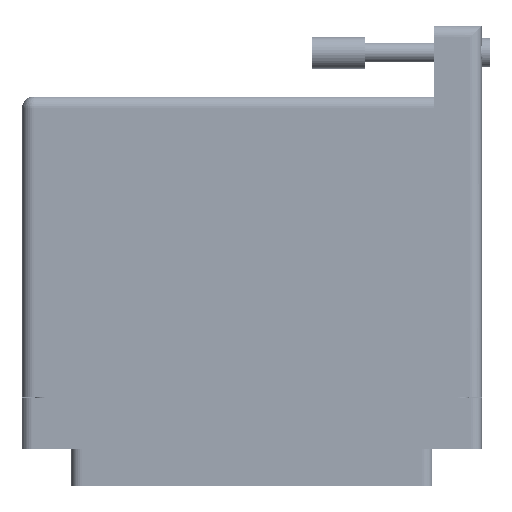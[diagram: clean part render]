
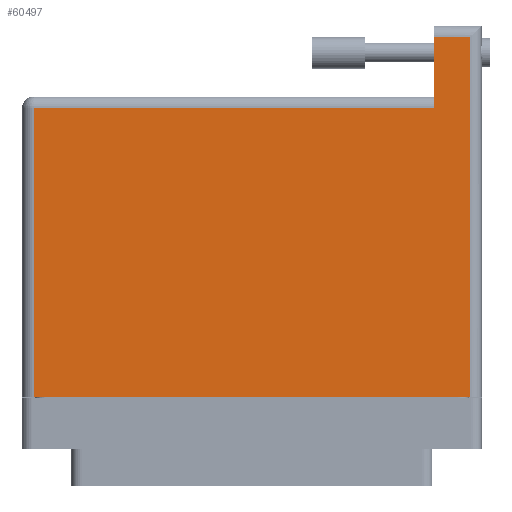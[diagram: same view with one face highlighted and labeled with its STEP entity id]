
A CAD part, front view. The second image highlights one B-rep face of the part: STEP entity #60497.
In plain terms, the highlighted face is planar.
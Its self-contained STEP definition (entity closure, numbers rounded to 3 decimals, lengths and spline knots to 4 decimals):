
#1102 = CARTESIAN_POINT ( 'NONE',  ( -1.359, 1.675, 0.617 ) ) ;
#1421 = LINE ( 'NONE', #1966, #57320 ) ;
#1966 = CARTESIAN_POINT ( 'NONE',  ( 1.079, 2.095, 0.617 ) ) ;
#2111 = FACE_OUTER_BOUND ( 'NONE', #41996, .T. ) ;
#6260 = VERTEX_POINT ( 'NONE', #32739 ) ;
#8278 = VERTEX_POINT ( 'NONE', #10705 ) ;
#10705 = CARTESIAN_POINT ( 'NONE',  ( -1.289, 1.605, 0.617 ) ) ;
#12804 = VECTOR ( 'NONE', #33574, 39.3701 ) ;
#13091 = DIRECTION ( 'NONE',  ( -1., 0., 0. ) ) ;
#14640 = VECTOR ( 'NONE', #34641, 39.3701 ) ;
#15283 = ORIENTED_EDGE ( 'NONE', *, *, #44509, .T. ) ;
#16572 = CARTESIAN_POINT ( 'NONE',  ( 1.289, -0.1, 0.617 ) ) ;
#18814 = ORIENTED_EDGE ( 'NONE', *, *, #52891, .T. ) ;
#19305 = VECTOR ( 'NONE', #24328, 39.3701 ) ;
#19913 = VERTEX_POINT ( 'NONE', #67257 ) ;
#22695 = LINE ( 'NONE', #39496, #19305 ) ;
#23028 = DIRECTION ( 'NONE',  ( 0., -1., 0. ) ) ;
#24328 = DIRECTION ( 'NONE',  ( 1., 0., 0. ) ) ;
#27177 = EDGE_CURVE ( 'NONE', #19913, #6260, #61173, .T. ) ;
#30400 = ORIENTED_EDGE ( 'NONE', *, *, #69777, .T. ) ;
#31073 = VERTEX_POINT ( 'NONE', #16572 ) ;
#32739 = CARTESIAN_POINT ( 'NONE',  ( 1.079, 2.025, 0.617 ) ) ;
#33574 = DIRECTION ( 'NONE',  ( 0., 1., 0. ) ) ;
#34641 = DIRECTION ( 'NONE',  ( -1., 0., 0. ) ) ;
#35326 = VERTEX_POINT ( 'NONE', #38211 ) ;
#38211 = CARTESIAN_POINT ( 'NONE',  ( 1.079, 1.605, 0.617 ) ) ;
#39496 = CARTESIAN_POINT ( 'NONE',  ( -1.359, -0.1, 0.617 ) ) ;
#39510 = CARTESIAN_POINT ( 'NONE',  ( 1.289, 2.095, 0.617 ) ) ;
#41996 = EDGE_LOOP ( 'NONE', ( #15283, #30400, #18814, #63349, #62808, #47853 ) ) ;
#44509 = EDGE_CURVE ( 'NONE', #35326, #8278, #68771, .T. ) ;
#45704 = CARTESIAN_POINT ( 'NONE',  ( -1.359, 2.025, 0.617 ) ) ;
#46667 = AXIS2_PLACEMENT_3D ( 'NONE', #1102, #49119, #59776 ) ;
#47790 = VERTEX_POINT ( 'NONE', #69207 ) ;
#47853 = ORIENTED_EDGE ( 'NONE', *, *, #51676, .T. ) ;
#49119 = DIRECTION ( 'NONE',  ( 0., 0., -1. ) ) ;
#49797 = VECTOR ( 'NONE', #56096, 39.3701 ) ;
#50446 = CARTESIAN_POINT ( 'NONE',  ( -1.289, -0.1, 0.617 ) ) ;
#51676 = EDGE_CURVE ( 'NONE', #6260, #35326, #1421, .T. ) ;
#52891 = EDGE_CURVE ( 'NONE', #47790, #31073, #22695, .T. ) ;
#54581 = PLANE ( 'NONE',  #46667 ) ;
#56096 = DIRECTION ( 'NONE',  ( 0., -1., 0. ) ) ;
#57320 = VECTOR ( 'NONE', #23028, 39.3701 ) ;
#59776 = DIRECTION ( 'NONE',  ( -1., 0., 0. ) ) ;
#60291 = VECTOR ( 'NONE', #13091, 39.3701 ) ;
#60497 = ADVANCED_FACE ( 'NONE', ( #2111 ), #54581, .F. ) ;
#61173 = LINE ( 'NONE', #45704, #60291 ) ;
#61660 = CARTESIAN_POINT ( 'NONE',  ( -1.359, 1.605, 0.617 ) ) ;
#62808 = ORIENTED_EDGE ( 'NONE', *, *, #27177, .T. ) ;
#63349 = ORIENTED_EDGE ( 'NONE', *, *, #68214, .T. ) ;
#66140 = LINE ( 'NONE', #39510, #12804 ) ;
#67257 = CARTESIAN_POINT ( 'NONE',  ( 1.289, 2.025, 0.617 ) ) ;
#67548 = LINE ( 'NONE', #50446, #49797 ) ;
#68214 = EDGE_CURVE ( 'NONE', #31073, #19913, #66140, .T. ) ;
#68771 = LINE ( 'NONE', #61660, #14640 ) ;
#69207 = CARTESIAN_POINT ( 'NONE',  ( -1.289, -0.1, 0.617 ) ) ;
#69777 = EDGE_CURVE ( 'NONE', #8278, #47790, #67548, .T. ) ;
